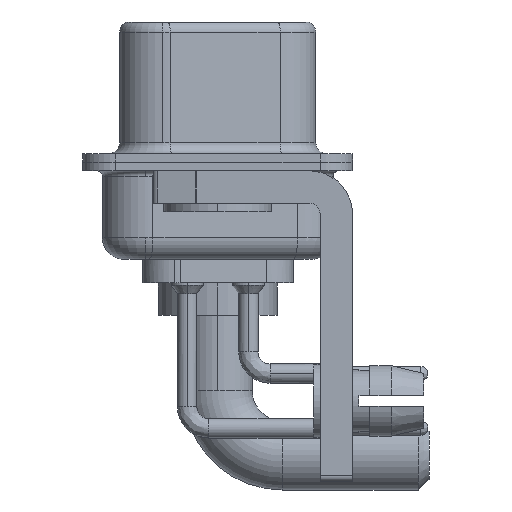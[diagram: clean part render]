
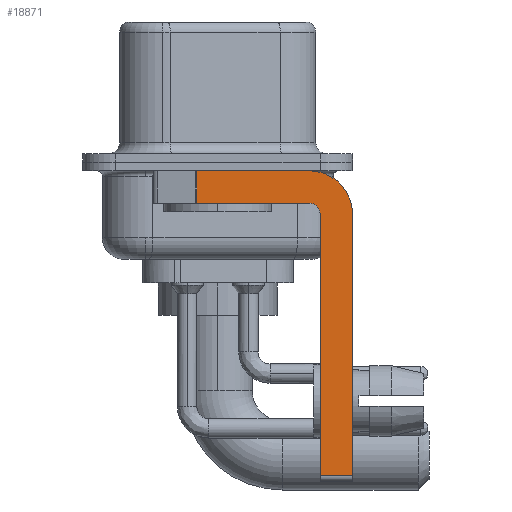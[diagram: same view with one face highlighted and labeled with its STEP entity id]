
A CAD part, left-side view. The second image highlights one B-rep face of the part: STEP entity #18871.
In plain terms, the highlighted planar face has unit normal (-1, 0, 0).
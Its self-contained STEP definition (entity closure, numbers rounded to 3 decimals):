
#496 = DIRECTION ( 'NONE',  ( 0., -1., 0. ) ) ;
#712 = CARTESIAN_POINT ( 'NONE',  ( -2.9, -4.25, -1.9 ) ) ;
#896 = DIRECTION ( 'NONE',  ( 0., -1., 0. ) ) ;
#1041 = CARTESIAN_POINT ( 'NONE',  ( -2.9, -4.25, -14.55 ) ) ;
#1873 = CARTESIAN_POINT ( 'NONE',  ( -2.9, -4.25, -2.4 ) ) ;
#1916 = ORIENTED_EDGE ( 'NONE', *, *, #19708, .F. ) ;
#1969 = DIRECTION ( 'NONE',  ( 0., 0., 1. ) ) ;
#1983 = ORIENTED_EDGE ( 'NONE', *, *, #26593, .F. ) ;
#2390 = VECTOR ( 'NONE', #496, 1000. ) ;
#2554 = VERTEX_POINT ( 'NONE', #25325 ) ;
#2731 = CARTESIAN_POINT ( 'NONE',  ( -2.9, -6.25, -14.55 ) ) ;
#3206 = DIRECTION ( 'NONE',  ( 0., 0., -1. ) ) ;
#3671 = EDGE_CURVE ( 'NONE', #2554, #14769, #9366, .T. ) ;
#3715 = ORIENTED_EDGE ( 'NONE', *, *, #3671, .T. ) ;
#3996 = LINE ( 'NONE', #14994, #11532 ) ;
#4250 = LINE ( 'NONE', #10982, #2390 ) ;
#4596 = AXIS2_PLACEMENT_3D ( 'NONE', #9234, #15797, #12971 ) ;
#4937 = CARTESIAN_POINT ( 'NONE',  ( -2.9, 0.978, -1.9 ) ) ;
#5010 = EDGE_CURVE ( 'NONE', #12954, #12054, #16922, .T. ) ;
#6555 = CIRCLE ( 'NONE', #26169, 0.5 ) ;
#7373 = DIRECTION ( 'NONE',  ( 1., 0., 0. ) ) ;
#7511 = CARTESIAN_POINT ( 'NONE',  ( -2.9, 0.978, -1.9 ) ) ;
#7849 = EDGE_CURVE ( 'NONE', #10465, #9058, #24927, .T. ) ;
#8112 = CARTESIAN_POINT ( 'NONE',  ( -2.9, -4.25, -0.4 ) ) ;
#8861 = CARTESIAN_POINT ( 'NONE',  ( -2.9, -6.25, -2.4 ) ) ;
#9058 = VERTEX_POINT ( 'NONE', #4937 ) ;
#9234 = CARTESIAN_POINT ( 'NONE',  ( -2.9, -4.25, -2.4 ) ) ;
#9366 = LINE ( 'NONE', #1041, #17442 ) ;
#10465 = VERTEX_POINT ( 'NONE', #18789 ) ;
#10715 = ORIENTED_EDGE ( 'NONE', *, *, #7849, .T. ) ;
#10982 = CARTESIAN_POINT ( 'NONE',  ( -2.9, 3., -0.4 ) ) ;
#11162 = LINE ( 'NONE', #8861, #23750 ) ;
#11397 = CARTESIAN_POINT ( 'NONE',  ( -2.9, -4.25, -2.4 ) ) ;
#11532 = VECTOR ( 'NONE', #1969, 1000. ) ;
#12054 = VERTEX_POINT ( 'NONE', #16896 ) ;
#12613 = EDGE_CURVE ( 'NONE', #2554, #14941, #3996, .T. ) ;
#12954 = VERTEX_POINT ( 'NONE', #8112 ) ;
#12971 = DIRECTION ( 'NONE',  ( 0., 0., -1. ) ) ;
#13690 = AXIS2_PLACEMENT_3D ( 'NONE', #11397, #7373, #15948 ) ;
#14321 = CARTESIAN_POINT ( 'NONE',  ( -2.9, -4.75, -2.4 ) ) ;
#14590 = VECTOR ( 'NONE', #3206, 1000. ) ;
#14769 = VERTEX_POINT ( 'NONE', #2731 ) ;
#14915 = VERTEX_POINT ( 'NONE', #20325 ) ;
#14941 = VERTEX_POINT ( 'NONE', #14321 ) ;
#14994 = CARTESIAN_POINT ( 'NONE',  ( -2.9, -4.75, -14.8 ) ) ;
#15501 = ORIENTED_EDGE ( 'NONE', *, *, #5010, .F. ) ;
#15524 = ORIENTED_EDGE ( 'NONE', *, *, #23133, .F. ) ;
#15797 = DIRECTION ( 'NONE',  ( 1., 0., 0. ) ) ;
#15948 = DIRECTION ( 'NONE',  ( 0., 0., -1. ) ) ;
#16325 = LINE ( 'NONE', #712, #21282 ) ;
#16896 = CARTESIAN_POINT ( 'NONE',  ( -2.9, -6.25, -2.4 ) ) ;
#16922 = CIRCLE ( 'NONE', #4596, 2. ) ;
#17442 = VECTOR ( 'NONE', #896, 1000. ) ;
#17683 = PLANE ( 'NONE',  #13690 ) ;
#18661 = ORIENTED_EDGE ( 'NONE', *, *, #12613, .F. ) ;
#18789 = CARTESIAN_POINT ( 'NONE',  ( -2.9, 0.978, -0.4 ) ) ;
#18871 = ADVANCED_FACE ( 'NONE', ( #22104 ), #17683, .F. ) ;
#19708 = EDGE_CURVE ( 'NONE', #12054, #14769, #11162, .T. ) ;
#20325 = CARTESIAN_POINT ( 'NONE',  ( -2.9, -4.25, -1.9 ) ) ;
#21282 = VECTOR ( 'NONE', #24583, 1000. ) ;
#21894 = DIRECTION ( 'NONE',  ( -1., 0., 0. ) ) ;
#22006 = DIRECTION ( 'NONE',  ( 0., 0., -1. ) ) ;
#22104 = FACE_OUTER_BOUND ( 'NONE', #27663, .T. ) ;
#23133 = EDGE_CURVE ( 'NONE', #10465, #12954, #4250, .T. ) ;
#23329 = ORIENTED_EDGE ( 'NONE', *, *, #24027, .F. ) ;
#23750 = VECTOR ( 'NONE', #22006, 1000. ) ;
#24027 = EDGE_CURVE ( 'NONE', #14941, #14915, #6555, .T. ) ;
#24583 = DIRECTION ( 'NONE',  ( 0., 1., 0. ) ) ;
#24927 = LINE ( 'NONE', #7511, #14590 ) ;
#25325 = CARTESIAN_POINT ( 'NONE',  ( -2.9, -4.75, -14.55 ) ) ;
#25742 = DIRECTION ( 'NONE',  ( 0., 0., 1. ) ) ;
#26169 = AXIS2_PLACEMENT_3D ( 'NONE', #1873, #21894, #25742 ) ;
#26593 = EDGE_CURVE ( 'NONE', #14915, #9058, #16325, .T. ) ;
#27663 = EDGE_LOOP ( 'NONE', ( #15524, #10715, #1983, #23329, #18661, #3715, #1916, #15501 ) ) ;
